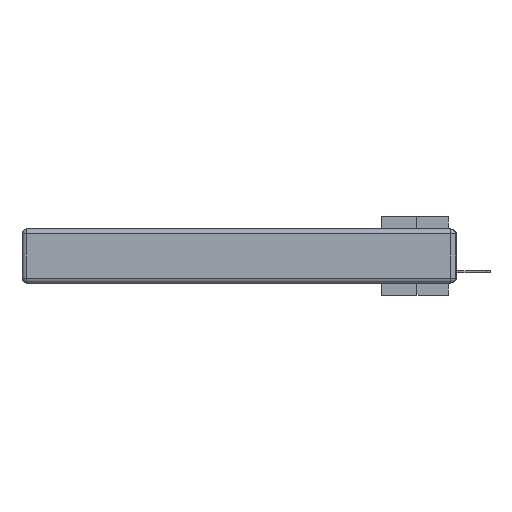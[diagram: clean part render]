
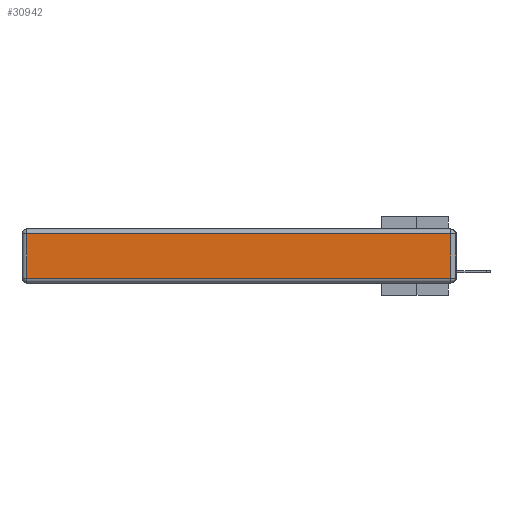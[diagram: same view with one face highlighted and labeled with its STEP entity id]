
A CAD part, left-side view. The second image highlights one B-rep face of the part: STEP entity #30942.
In plain terms, the highlighted planar face has unit normal (-1, 0, 0).
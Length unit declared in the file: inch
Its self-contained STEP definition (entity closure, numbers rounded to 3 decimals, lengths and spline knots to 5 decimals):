
#1423 = DIRECTION ( 'NONE',  ( 0., 0., 1. ) ) ;
#3154 = CARTESIAN_POINT ( 'NONE',  ( 0., 0., -0.343 ) ) ;
#3548 = EDGE_CURVE ( 'NONE', #13454, #31572, #27819, .T. ) ;
#3710 = CARTESIAN_POINT ( 'NONE',  ( 0., 2.72, -0.313 ) ) ;
#4731 = LINE ( 'NONE', #23807, #30804 ) ;
#7302 = VECTOR ( 'NONE', #31127, 39.37008 ) ;
#9972 = PLANE ( 'NONE',  #31983 ) ;
#10129 = VECTOR ( 'NONE', #24637, 39.37008 ) ;
#13207 = ORIENTED_EDGE ( 'NONE', *, *, #31028, .T. ) ;
#13454 = VERTEX_POINT ( 'NONE', #3710 ) ;
#14753 = CARTESIAN_POINT ( 'NONE',  ( 0., 2.72, -0.03 ) ) ;
#15969 = DIRECTION ( 'NONE',  ( 0., 0., 1. ) ) ;
#17906 = EDGE_CURVE ( 'NONE', #31572, #18918, #4731, .T. ) ;
#18198 = CARTESIAN_POINT ( 'NONE',  ( 0., 2.75, -0.03 ) ) ;
#18918 = VERTEX_POINT ( 'NONE', #20577 ) ;
#19287 = FACE_OUTER_BOUND ( 'NONE', #20297, .T. ) ;
#20297 = EDGE_LOOP ( 'NONE', ( #26019, #24373, #13207, #35947 ) ) ;
#20577 = CARTESIAN_POINT ( 'NONE',  ( 0., 0.03, -0.03 ) ) ;
#23558 = LINE ( 'NONE', #24161, #39053 ) ;
#23807 = CARTESIAN_POINT ( 'NONE',  ( 0., 0.03, -0.343 ) ) ;
#23957 = DIRECTION ( 'NONE',  ( 0., 0., -1. ) ) ;
#24161 = CARTESIAN_POINT ( 'NONE',  ( 0., 2.72, -0.343 ) ) ;
#24373 = ORIENTED_EDGE ( 'NONE', *, *, #17906, .T. ) ;
#24637 = DIRECTION ( 'NONE',  ( 0., 1., 0. ) ) ;
#26019 = ORIENTED_EDGE ( 'NONE', *, *, #3548, .T. ) ;
#26321 = EDGE_CURVE ( 'NONE', #40948, #13454, #23558, .T. ) ;
#27290 = CARTESIAN_POINT ( 'NONE',  ( 0., 0.03, -0.313 ) ) ;
#27819 = LINE ( 'NONE', #28008, #7302 ) ;
#28008 = CARTESIAN_POINT ( 'NONE',  ( 0., 0., -0.313 ) ) ;
#30804 = VECTOR ( 'NONE', #1423, 39.37008 ) ;
#30942 = ADVANCED_FACE ( 'NONE', ( #19287 ), #9972, .T. ) ;
#31028 = EDGE_CURVE ( 'NONE', #18918, #40948, #34376, .T. ) ;
#31127 = DIRECTION ( 'NONE',  ( 0., -1., 0. ) ) ;
#31572 = VERTEX_POINT ( 'NONE', #27290 ) ;
#31983 = AXIS2_PLACEMENT_3D ( 'NONE', #3154, #38165, #15969 ) ;
#34376 = LINE ( 'NONE', #18198, #10129 ) ;
#35947 = ORIENTED_EDGE ( 'NONE', *, *, #26321, .T. ) ;
#38165 = DIRECTION ( 'NONE',  ( -1., 0., 0. ) ) ;
#39053 = VECTOR ( 'NONE', #23957, 39.37008 ) ;
#40948 = VERTEX_POINT ( 'NONE', #14753 ) ;
